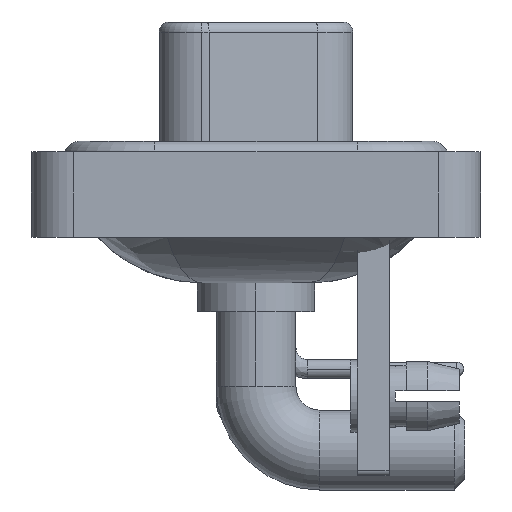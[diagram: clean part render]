
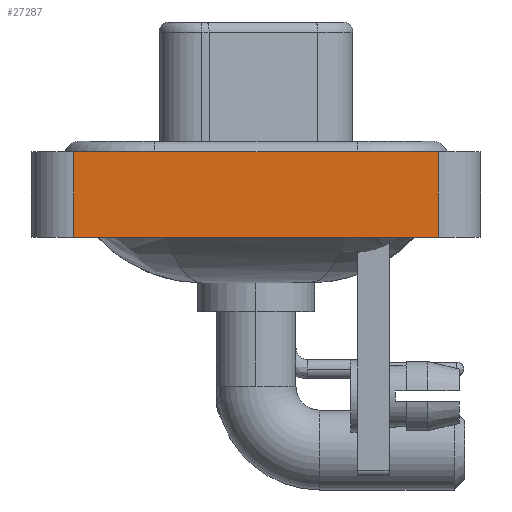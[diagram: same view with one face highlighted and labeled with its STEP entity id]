
A CAD part, left-side view. The second image highlights one B-rep face of the part: STEP entity #27287.
In plain terms, the highlighted planar face has unit normal (-1, 0, 0).
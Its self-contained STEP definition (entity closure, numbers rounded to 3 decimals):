
#726 = CARTESIAN_POINT ( 'NONE',  ( -7.35, -8.55, -3.6 ) ) ;
#1272 = DIRECTION ( 'NONE',  ( 0., -1., 0. ) ) ;
#2085 = EDGE_CURVE ( 'NONE', #19009, #22519, #7336, .T. ) ;
#2541 = CARTESIAN_POINT ( 'NONE',  ( -7.35, 8.55, -3.6 ) ) ;
#2989 = PLANE ( 'NONE',  #14411 ) ;
#3339 = CARTESIAN_POINT ( 'NONE',  ( -7.35, 8.55, 0.4 ) ) ;
#3638 = VECTOR ( 'NONE', #1272, 1000. ) ;
#4317 = LINE ( 'NONE', #10938, #20929 ) ;
#4697 = ORIENTED_EDGE ( 'NONE', *, *, #18496, .F. ) ;
#4939 = DIRECTION ( 'NONE',  ( -1., 0., 0. ) ) ;
#5626 = EDGE_CURVE ( 'NONE', #19009, #24058, #13160, .T. ) ;
#6505 = VERTEX_POINT ( 'NONE', #28953 ) ;
#6656 = ORIENTED_EDGE ( 'NONE', *, *, #26148, .T. ) ;
#7336 = LINE ( 'NONE', #2541, #25002 ) ;
#8785 = DIRECTION ( 'NONE',  ( 0., -1., 0. ) ) ;
#10938 = CARTESIAN_POINT ( 'NONE',  ( -7.35, -8.55, -3.6 ) ) ;
#11056 = CARTESIAN_POINT ( 'NONE',  ( -7.35, -8.55, -3.6 ) ) ;
#12677 = ORIENTED_EDGE ( 'NONE', *, *, #5626, .T. ) ;
#12700 = LINE ( 'NONE', #21825, #3638 ) ;
#13160 = LINE ( 'NONE', #11056, #25592 ) ;
#14411 = AXIS2_PLACEMENT_3D ( 'NONE', #726, #4939, #25198 ) ;
#16510 = DIRECTION ( 'NONE',  ( 0., 0., 1. ) ) ;
#18496 = EDGE_CURVE ( 'NONE', #22519, #6505, #12700, .T. ) ;
#19009 = VERTEX_POINT ( 'NONE', #28054 ) ;
#20929 = VECTOR ( 'NONE', #29349, 1000. ) ;
#21303 = CARTESIAN_POINT ( 'NONE',  ( -7.35, -8.55, -3.6 ) ) ;
#21825 = CARTESIAN_POINT ( 'NONE',  ( -7.35, -8.55, 0.4 ) ) ;
#21973 = ORIENTED_EDGE ( 'NONE', *, *, #2085, .F. ) ;
#22519 = VERTEX_POINT ( 'NONE', #3339 ) ;
#23550 = FACE_OUTER_BOUND ( 'NONE', #29449, .T. ) ;
#24058 = VERTEX_POINT ( 'NONE', #21303 ) ;
#25002 = VECTOR ( 'NONE', #16510, 1000. ) ;
#25198 = DIRECTION ( 'NONE',  ( 0., 0., 1. ) ) ;
#25592 = VECTOR ( 'NONE', #8785, 1000. ) ;
#26148 = EDGE_CURVE ( 'NONE', #24058, #6505, #4317, .T. ) ;
#27287 = ADVANCED_FACE ( 'NONE', ( #23550 ), #2989, .T. ) ;
#28054 = CARTESIAN_POINT ( 'NONE',  ( -7.35, 8.55, -3.6 ) ) ;
#28953 = CARTESIAN_POINT ( 'NONE',  ( -7.35, -8.55, 0.4 ) ) ;
#29349 = DIRECTION ( 'NONE',  ( 0., 0., 1. ) ) ;
#29449 = EDGE_LOOP ( 'NONE', ( #6656, #4697, #21973, #12677 ) ) ;
